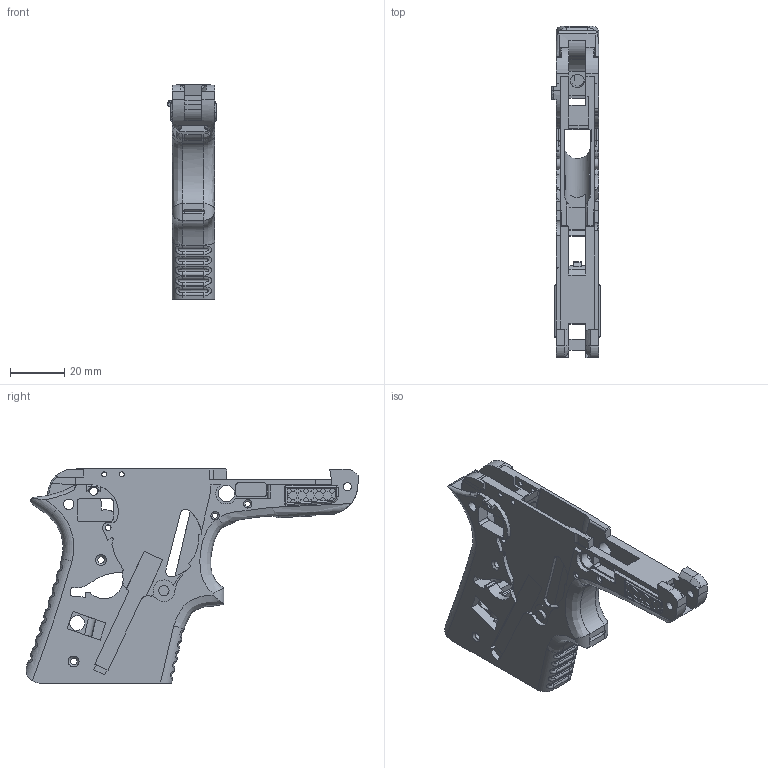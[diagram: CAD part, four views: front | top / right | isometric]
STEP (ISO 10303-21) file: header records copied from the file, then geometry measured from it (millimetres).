
FILE_DESCRIPTION(/* description */ (''),/* implementation_level */ '2;1');
FILE_NAME(/* name */ '21a-frame-final.step',/* time_stamp */ '2021-11-09T19:51:52-08:00',/* author */ (''),/* organization */ (''),/* preprocessor_version */ 'ST-DEVELOPER v18.1',/* originating_system */ 'Autodesk Translation Framework v10.10.0.1391',/* authorisation */ '');
FILE_SCHEMA (('AUTOMOTIVE_DESIGN { 1 0 10303 214 3 1 1 }'));
Products named in the file (1): 21a-frame-final
Bounding box: 17.71 x 122.46 x 78.94 mm (x, y, z)
Volume: 40893.6 mm3; surface area: 26142.8 mm2
Topology: 1 solids, 1 shells, 1540 faces, 4366 edges, 2851 vertices
Faces by surface type: bspline 750, plane 537, cylinder 218, torus 18, cone 15, sphere 2
Full cylindrical faces by diameter (mm): 1.8 x4, 2.05 x2, 2.1 x2, 2.14 x2, 2.5 x3, 2.98 x2, 3 x2, 3.8 x4, 5 x1, 5.5 x1, 6.1 x2, 8.7 x1
Entity records: 59809 total; most frequent: CARTESIAN_POINT 24613, ORIENTED_EDGE 8712, DIRECTION 4933, EDGE_CURVE 4356, VERTEX_POINT 2851, LINE 2261, VECTOR 2261, EDGE_LOOP 1641
